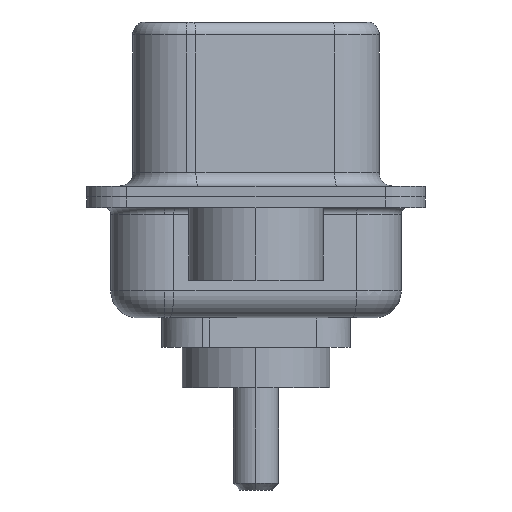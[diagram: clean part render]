
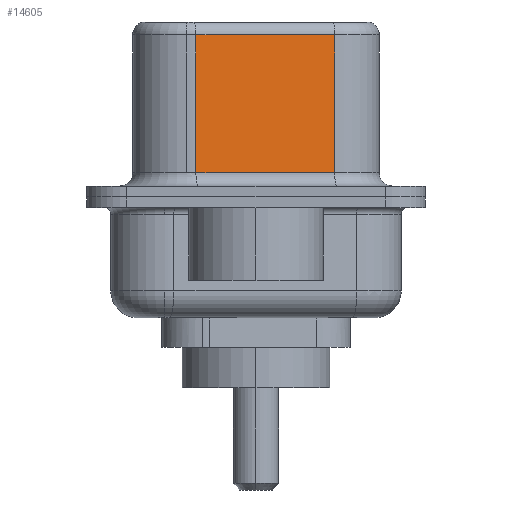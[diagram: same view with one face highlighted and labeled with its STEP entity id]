
A CAD part, left-side view. The second image highlights one B-rep face of the part: STEP entity #14605.
In plain terms, the highlighted planar face has unit normal (-0.985, -0.174, 0).
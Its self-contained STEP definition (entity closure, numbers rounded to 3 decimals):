
#24 = EDGE_CURVE ( 'NONE', #1645, #12772, #10058, .T. ) ;
#1117 = DIRECTION ( 'NONE',  ( -0.174, 0.985, 0. ) ) ;
#1645 = VERTEX_POINT ( 'NONE', #13040 ) ;
#1819 = VECTOR ( 'NONE', #2093, 1000. ) ;
#1831 = FACE_OUTER_BOUND ( 'NONE', #12486, .T. ) ;
#1865 = ORIENTED_EDGE ( 'NONE', *, *, #24, .T. ) ;
#2076 = EDGE_CURVE ( 'NONE', #4974, #12772, #11018, .T. ) ;
#2093 = DIRECTION ( 'NONE',  ( 0., 0., -1. ) ) ;
#2354 = ORIENTED_EDGE ( 'NONE', *, *, #11357, .T. ) ;
#2854 = CARTESIAN_POINT ( 'NONE',  ( 4.565, -2.927, 0.9 ) ) ;
#2952 = CARTESIAN_POINT ( 'NONE',  ( 4.565, -2.927, 0.9 ) ) ;
#3194 = DIRECTION ( 'NONE',  ( -0.174, 0.985, 0. ) ) ;
#3196 = VECTOR ( 'NONE', #6567, 1000. ) ;
#4039 = VECTOR ( 'NONE', #10253, 1000. ) ;
#4974 = VERTEX_POINT ( 'NONE', #8022 ) ;
#5043 = ORIENTED_EDGE ( 'NONE', *, *, #2076, .F. ) ;
#6029 = ORIENTED_EDGE ( 'NONE', *, *, #6781, .T. ) ;
#6567 = DIRECTION ( 'NONE',  ( 0., 0., -1. ) ) ;
#6710 = AXIS2_PLACEMENT_3D ( 'NONE', #9160, #10402, #3194 ) ;
#6728 = LINE ( 'NONE', #6896, #3196 ) ;
#6781 = EDGE_CURVE ( 'NONE', #11797, #1645, #6728, .T. ) ;
#6896 = CARTESIAN_POINT ( 'NONE',  ( 3.655, 2.233, 6.52 ) ) ;
#7774 = CARTESIAN_POINT ( 'NONE',  ( 4.565, -2.927, 6.52 ) ) ;
#7972 = PLANE ( 'NONE',  #6710 ) ;
#8022 = CARTESIAN_POINT ( 'NONE',  ( 4.565, -2.927, 6.02 ) ) ;
#8516 = CARTESIAN_POINT ( 'NONE',  ( 3.655, 2.233, 6.02 ) ) ;
#9160 = CARTESIAN_POINT ( 'NONE',  ( 4.565, -2.927, 6.52 ) ) ;
#9491 = CARTESIAN_POINT ( 'NONE',  ( 4.565, -2.927, 6.02 ) ) ;
#10058 = LINE ( 'NONE', #2854, #4039 ) ;
#10253 = DIRECTION ( 'NONE',  ( 0.174, -0.985, 0. ) ) ;
#10402 = DIRECTION ( 'NONE',  ( 0.985, 0.174, 0. ) ) ;
#11018 = LINE ( 'NONE', #7774, #1819 ) ;
#11357 = EDGE_CURVE ( 'NONE', #4974, #11797, #15203, .T. ) ;
#11797 = VERTEX_POINT ( 'NONE', #8516 ) ;
#11982 = VECTOR ( 'NONE', #1117, 1000. ) ;
#12486 = EDGE_LOOP ( 'NONE', ( #5043, #2354, #6029, #1865 ) ) ;
#12772 = VERTEX_POINT ( 'NONE', #2952 ) ;
#13040 = CARTESIAN_POINT ( 'NONE',  ( 3.655, 2.233, 0.9 ) ) ;
#14605 = ADVANCED_FACE ( 'NONE', ( #1831 ), #7972, .F. ) ;
#15203 = LINE ( 'NONE', #9491, #11982 ) ;
